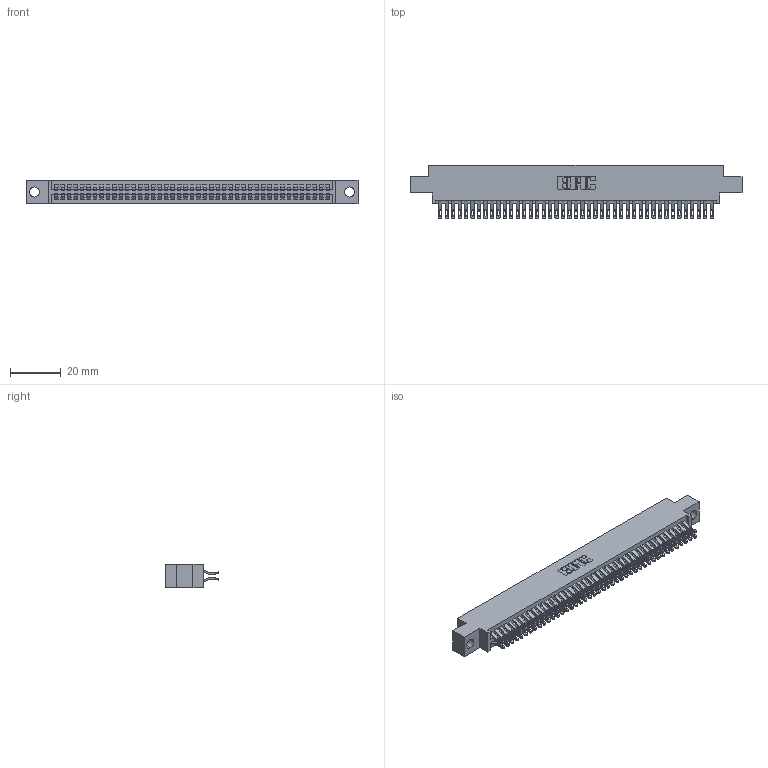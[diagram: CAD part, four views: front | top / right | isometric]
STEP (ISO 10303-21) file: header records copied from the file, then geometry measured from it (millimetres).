
FILE_DESCRIPTION (( 'STEP AP203' ), '1' );
FILE_NAME ('395-086-555-804.STEP', '2021-06-17T09:03:56', ( '' ), ( '' ), 'SwSTEP 2.0', 'SolidWorks 2020', '' );
FILE_SCHEMA (( 'CONFIG_CONTROL_DESIGN' ));
Length unit declared in the file: inch
Products named in the file (3): 345-292-001_555 Tail; 395-086-555-804; 345 Part_0.170 Offset - 0.156 Dia-TI
Assembly tree (87 placements, depth 2):
  395-086-555-804
    345 Part_0.170 Offset - 0.156 Dia-TI
    345-292-001_555 Tail  x86
Bounding box: 130.43 x 21.13 x 9.4 mm (x, y, z)
Volume: 12709.4 mm3; surface area: 19668.7 mm2
Topology: 87 solids, 87 shells, 4960 faces, 15611 edges, 10406 vertices
Faces by surface type: plane 2764, cylinder 2196
Entity records: 34481 total; most frequent: CARTESIAN_POINT 5820, ORIENTED_EDGE 5722, DIRECTION 5097, EDGE_CURVE 2861, VECTOR 2537, LINE 2537, VERTEX_POINT 1906, AXIS2_PLACEMENT_3D 1280
